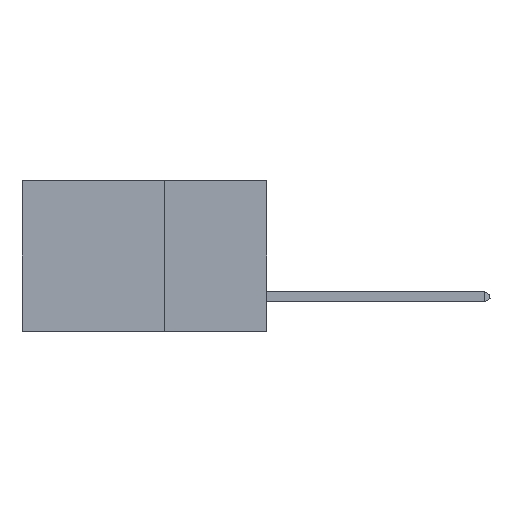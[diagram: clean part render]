
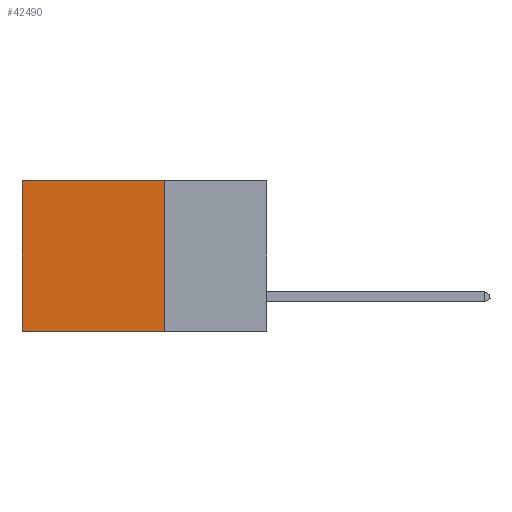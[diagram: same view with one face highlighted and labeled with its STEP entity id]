
A CAD part, left-side view. The second image highlights one B-rep face of the part: STEP entity #42490.
In plain terms, the highlighted planar face has unit normal (-1, 0, 0).
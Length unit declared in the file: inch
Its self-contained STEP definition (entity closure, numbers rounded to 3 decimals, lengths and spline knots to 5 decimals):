
#445 = EDGE_CURVE ( 'NONE', #23132, #5669, #24952, .T. ) ;
#765 = DIRECTION ( 'NONE',  ( 0., 0., -1. ) ) ;
#852 = CARTESIAN_POINT ( 'NONE',  ( 0.2875, 0.25, -0.37 ) ) ;
#1284 = ORIENTED_EDGE ( 'NONE', *, *, #23783, .T. ) ;
#2924 = ORIENTED_EDGE ( 'NONE', *, *, #445, .T. ) ;
#3661 = DIRECTION ( 'NONE',  ( 0., 1., 0. ) ) ;
#3949 = LINE ( 'NONE', #5339, #33695 ) ;
#5339 = CARTESIAN_POINT ( 'NONE',  ( 0.2875, 0.25, 0. ) ) ;
#5669 = VERTEX_POINT ( 'NONE', #25680 ) ;
#6537 = FACE_OUTER_BOUND ( 'NONE', #11080, .T. ) ;
#6539 = VERTEX_POINT ( 'NONE', #31539 ) ;
#7040 = CARTESIAN_POINT ( 'NONE',  ( 0.2875, 0.25, 0. ) ) ;
#10157 = ORIENTED_EDGE ( 'NONE', *, *, #32307, .F. ) ;
#10640 = DIRECTION ( 'NONE',  ( 1., 0., 0. ) ) ;
#11080 = EDGE_LOOP ( 'NONE', ( #2924, #32178, #10157, #1284 ) ) ;
#11847 = LINE ( 'NONE', #7040, #43753 ) ;
#16924 = DIRECTION ( 'NONE',  ( 0., 0., -1. ) ) ;
#17989 = VECTOR ( 'NONE', #3661, 39.37008 ) ;
#20744 = CARTESIAN_POINT ( 'NONE',  ( 0.2875, 0.25, 0. ) ) ;
#23132 = VERTEX_POINT ( 'NONE', #41747 ) ;
#23783 = EDGE_CURVE ( 'NONE', #6539, #23132, #11847, .T. ) ;
#24323 = CARTESIAN_POINT ( 'NONE',  ( 0.2875, 0.25, -0.37 ) ) ;
#24952 = LINE ( 'NONE', #41849, #43018 ) ;
#25680 = CARTESIAN_POINT ( 'NONE',  ( 0.2875, 0.6, -0.37 ) ) ;
#27207 = VERTEX_POINT ( 'NONE', #24323 ) ;
#31539 = CARTESIAN_POINT ( 'NONE',  ( 0.2875, 0.25, 0. ) ) ;
#32057 = DIRECTION ( 'NONE',  ( 0., 0., -1. ) ) ;
#32178 = ORIENTED_EDGE ( 'NONE', *, *, #43759, .F. ) ;
#32271 = DIRECTION ( 'NONE',  ( 0., 1., 0. ) ) ;
#32307 = EDGE_CURVE ( 'NONE', #6539, #27207, #3949, .T. ) ;
#33695 = VECTOR ( 'NONE', #32057, 39.37008 ) ;
#36894 = AXIS2_PLACEMENT_3D ( 'NONE', #20744, #10640, #16924 ) ;
#37313 = PLANE ( 'NONE',  #36894 ) ;
#38818 = LINE ( 'NONE', #852, #17989 ) ;
#41747 = CARTESIAN_POINT ( 'NONE',  ( 0.2875, 0.6, 0. ) ) ;
#41849 = CARTESIAN_POINT ( 'NONE',  ( 0.2875, 0.6, 0. ) ) ;
#42490 = ADVANCED_FACE ( 'NONE', ( #6537 ), #37313, .F. ) ;
#43018 = VECTOR ( 'NONE', #765, 39.37008 ) ;
#43753 = VECTOR ( 'NONE', #32271, 39.37008 ) ;
#43759 = EDGE_CURVE ( 'NONE', #27207, #5669, #38818, .T. ) ;
